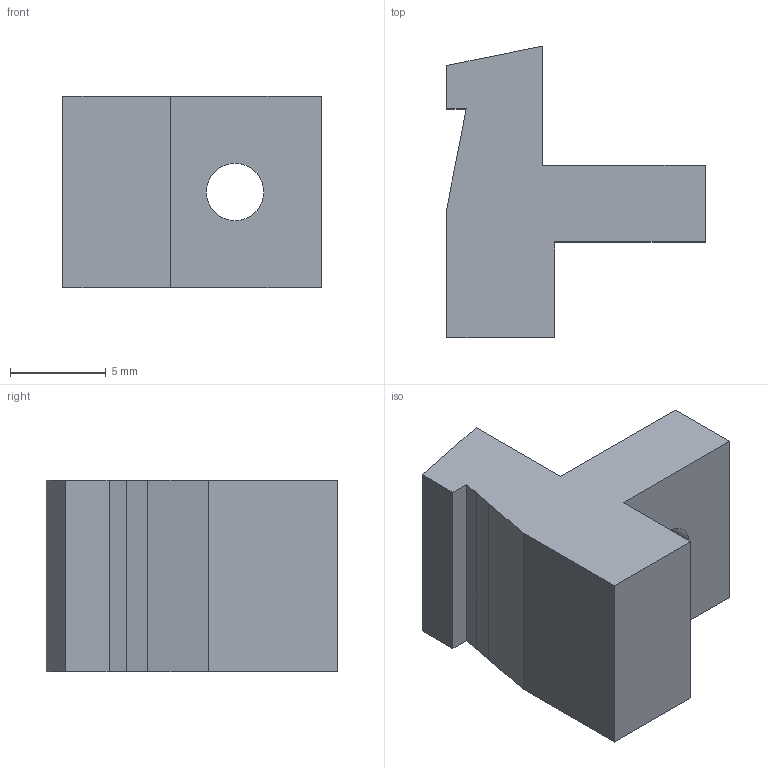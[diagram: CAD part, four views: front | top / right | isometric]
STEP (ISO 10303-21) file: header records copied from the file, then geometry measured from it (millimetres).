
FILE_DESCRIPTION(('STEP AP214'),'1');
FILE_NAME('Mod9 Feed Ramp Final.stp','2020-09-28T22:45:43',(' '),(' '),'Spatial InterOp 3D',' ',' ');
FILE_SCHEMA(('AUTOMOTIVE_DESIGN { 1 0 10303 214 1 1 1 1 }'));
Length unit declared in the file: metre
Products named in the file (1): ASM Body
Bounding box: 13.5 x 15.24 x 10 mm (x, y, z)
Volume: 1026.5 mm3; surface area: 810.8 mm2
Topology: 1 solids, 1 shells, 19 faces, 49 edges, 32 vertices
Faces by surface type: plane 15, cylinder 2, cone 2
Entity records: 602 total; most frequent: CARTESIAN_POINT 101, ORIENTED_EDGE 98, DIRECTION 95, EDGE_CURVE 49, LINE 43, VECTOR 43, VERTEX_POINT 32, AXIS2_PLACEMENT_3D 26
